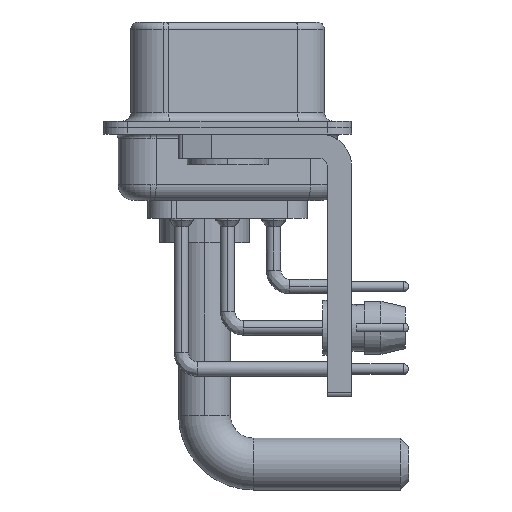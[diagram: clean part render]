
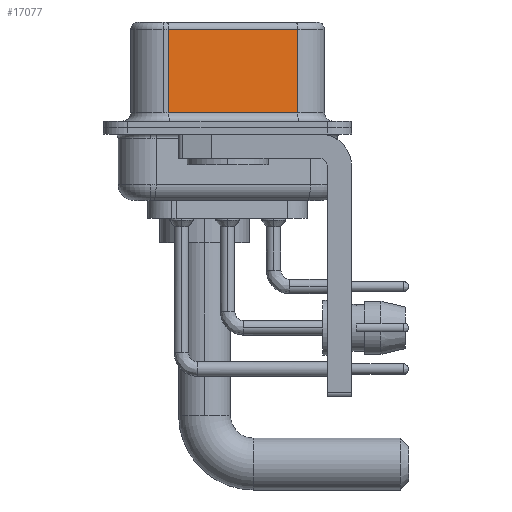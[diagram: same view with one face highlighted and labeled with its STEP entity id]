
A CAD part, left-side view. The second image highlights one B-rep face of the part: STEP entity #17077.
In plain terms, the highlighted planar face has unit normal (-0.985, -0.174, 0).
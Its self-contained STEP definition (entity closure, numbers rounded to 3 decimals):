
#1995 = ORIENTED_EDGE ( 'NONE', *, *, #28743, .T. ) ;
#3249 = ORIENTED_EDGE ( 'NONE', *, *, #19248, .T. ) ;
#5763 = CARTESIAN_POINT ( 'NONE',  ( 5.132, -4.322, 6.02 ) ) ;
#5823 = DIRECTION ( 'NONE',  ( 0.174, -0.985, 0. ) ) ;
#5998 = EDGE_CURVE ( 'NONE', #35378, #21961, #30341, .T. ) ;
#8609 = LINE ( 'NONE', #25103, #35150 ) ;
#10207 = CARTESIAN_POINT ( 'NONE',  ( 3.73, 3.628, 6.02 ) ) ;
#10812 = VECTOR ( 'NONE', #5823, 1000. ) ;
#10853 = VERTEX_POINT ( 'NONE', #10207 ) ;
#12096 = VECTOR ( 'NONE', #15400, 1000. ) ;
#15400 = DIRECTION ( 'NONE',  ( -0.174, 0.985, 0. ) ) ;
#17077 = ADVANCED_FACE ( 'NONE', ( #37050 ), #30991, .F. ) ;
#18872 = DIRECTION ( 'NONE',  ( 0., 0., -1. ) ) ;
#19248 = EDGE_CURVE ( 'NONE', #10853, #35378, #37362, .T. ) ;
#19563 = VERTEX_POINT ( 'NONE', #38963 ) ;
#20922 = EDGE_CURVE ( 'NONE', #19563, #21961, #8609, .T. ) ;
#21954 = DIRECTION ( 'NONE',  ( -0.174, 0.985, 0. ) ) ;
#21961 = VERTEX_POINT ( 'NONE', #33194 ) ;
#24950 = EDGE_LOOP ( 'NONE', ( #35086, #1995, #3249, #35703 ) ) ;
#25103 = CARTESIAN_POINT ( 'NONE',  ( 5.132, -4.322, 6.52 ) ) ;
#25160 = CARTESIAN_POINT ( 'NONE',  ( 5.132, -4.322, 6.52 ) ) ;
#27514 = CARTESIAN_POINT ( 'NONE',  ( 5.132, -4.322, 0.9 ) ) ;
#28291 = DIRECTION ( 'NONE',  ( 0., 0., -1. ) ) ;
#28743 = EDGE_CURVE ( 'NONE', #19563, #10853, #30875, .T. ) ;
#29224 = AXIS2_PLACEMENT_3D ( 'NONE', #25160, #34420, #21954 ) ;
#29869 = CARTESIAN_POINT ( 'NONE',  ( 3.73, 3.628, 0.9 ) ) ;
#30341 = LINE ( 'NONE', #27514, #10812 ) ;
#30875 = LINE ( 'NONE', #5763, #12096 ) ;
#30991 = PLANE ( 'NONE',  #29224 ) ;
#33194 = CARTESIAN_POINT ( 'NONE',  ( 5.132, -4.322, 0.9 ) ) ;
#33543 = CARTESIAN_POINT ( 'NONE',  ( 3.73, 3.628, 6.52 ) ) ;
#33836 = VECTOR ( 'NONE', #28291, 1000. ) ;
#34420 = DIRECTION ( 'NONE',  ( 0.985, 0.174, 0. ) ) ;
#35086 = ORIENTED_EDGE ( 'NONE', *, *, #20922, .F. ) ;
#35150 = VECTOR ( 'NONE', #18872, 1000. ) ;
#35378 = VERTEX_POINT ( 'NONE', #29869 ) ;
#35703 = ORIENTED_EDGE ( 'NONE', *, *, #5998, .T. ) ;
#37050 = FACE_OUTER_BOUND ( 'NONE', #24950, .T. ) ;
#37362 = LINE ( 'NONE', #33543, #33836 ) ;
#38963 = CARTESIAN_POINT ( 'NONE',  ( 5.132, -4.322, 6.02 ) ) ;
